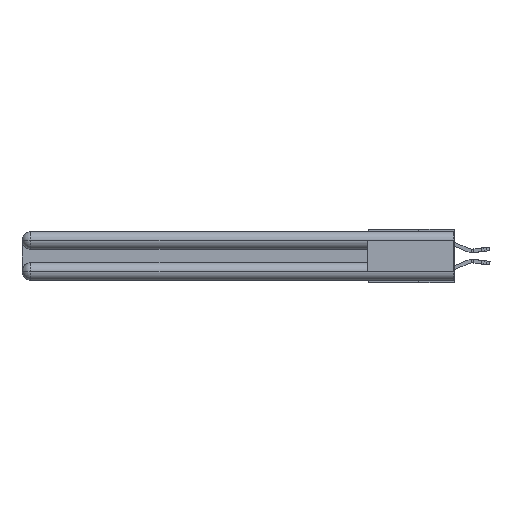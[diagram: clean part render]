
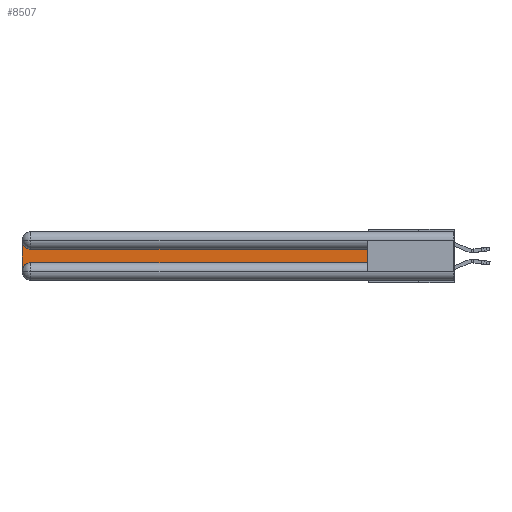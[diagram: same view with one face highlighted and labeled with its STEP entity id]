
A CAD part, left-side view. The second image highlights one B-rep face of the part: STEP entity #8507.
In plain terms, the highlighted planar face has unit normal (-1, 0, 0).
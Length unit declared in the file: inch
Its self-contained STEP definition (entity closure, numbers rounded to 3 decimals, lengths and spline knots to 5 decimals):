
#123 = CARTESIAN_POINT ( 'NONE',  ( 0.075, 3., -0.2175 ) ) ;
#2164 = LINE ( 'NONE', #10606, #26529 ) ;
#2321 = FACE_OUTER_BOUND ( 'NONE', #27542, .T. ) ;
#2388 = ORIENTED_EDGE ( 'NONE', *, *, #28134, .T. ) ;
#3236 = LINE ( 'NONE', #13092, #13530 ) ;
#3814 = CARTESIAN_POINT ( 'NONE',  ( 0.075, 2.94, -0.2775 ) ) ;
#4201 = EDGE_CURVE ( 'NONE', #28403, #14134, #21921, .T. ) ;
#6936 = CARTESIAN_POINT ( 'NONE',  ( 0.075, 2.94, -0.0625 ) ) ;
#6988 = AXIS2_PLACEMENT_3D ( 'NONE', #6936, #8967, #22307 ) ;
#7721 = ORIENTED_EDGE ( 'NONE', *, *, #15233, .T. ) ;
#8307 = VERTEX_POINT ( 'NONE', #20167 ) ;
#8507 = ADVANCED_FACE ( 'NONE', ( #2321 ), #12040, .F. ) ;
#8967 = DIRECTION ( 'NONE',  ( 1., 0., 0. ) ) ;
#9269 = AXIS2_PLACEMENT_3D ( 'NONE', #10018, #27425, #23078 ) ;
#10018 = CARTESIAN_POINT ( 'NONE',  ( 0.075, 3., -0.1225 ) ) ;
#10606 = CARTESIAN_POINT ( 'NONE',  ( 0.075, 0.6, -0.1225 ) ) ;
#11054 = CARTESIAN_POINT ( 'NONE',  ( 0.075, 0.6, -0.1225 ) ) ;
#12040 = PLANE ( 'NONE',  #9269 ) ;
#12139 = DIRECTION ( 'NONE',  ( 0., 0., 1. ) ) ;
#13092 = CARTESIAN_POINT ( 'NONE',  ( 0.075, 0.6, -0.2175 ) ) ;
#13530 = VECTOR ( 'NONE', #26231, 39.37008 ) ;
#13618 = ORIENTED_EDGE ( 'NONE', *, *, #28012, .T. ) ;
#14134 = VERTEX_POINT ( 'NONE', #11054 ) ;
#15233 = EDGE_CURVE ( 'NONE', #26937, #8307, #15254, .T. ) ;
#15254 = LINE ( 'NONE', #123, #21451 ) ;
#16101 = VECTOR ( 'NONE', #12139, 39.37008 ) ;
#16615 = DIRECTION ( 'NONE',  ( 1., 0., 0. ) ) ;
#17108 = ORIENTED_EDGE ( 'NONE', *, *, #18627, .T. ) ;
#17190 = CARTESIAN_POINT ( 'NONE',  ( 0.075, 0.6, -0.2175 ) ) ;
#17533 = VERTEX_POINT ( 'NONE', #18312 ) ;
#17835 = CIRCLE ( 'NONE', #24582, 0.06 ) ;
#18312 = CARTESIAN_POINT ( 'NONE',  ( 0.075, 2.94, -0.1225 ) ) ;
#18627 = EDGE_CURVE ( 'NONE', #14134, #17533, #2164, .T. ) ;
#18814 = ORIENTED_EDGE ( 'NONE', *, *, #4201, .T. ) ;
#20167 = CARTESIAN_POINT ( 'NONE',  ( 0.075, 3., -0.2775 ) ) ;
#21005 = DIRECTION ( 'NONE',  ( 0., 0., -1. ) ) ;
#21451 = VECTOR ( 'NONE', #22004, 39.37008 ) ;
#21921 = LINE ( 'NONE', #17190, #16101 ) ;
#22004 = DIRECTION ( 'NONE',  ( 0., 0., -1. ) ) ;
#22307 = DIRECTION ( 'NONE',  ( 0., 0., -1. ) ) ;
#22406 = VERTEX_POINT ( 'NONE', #24631 ) ;
#22984 = EDGE_CURVE ( 'NONE', #8307, #22406, #17835, .T. ) ;
#23078 = DIRECTION ( 'NONE',  ( 0., 0., -1. ) ) ;
#23927 = CARTESIAN_POINT ( 'NONE',  ( 0.075, 3., -0.0625 ) ) ;
#24182 = CIRCLE ( 'NONE', #6988, 0.06 ) ;
#24582 = AXIS2_PLACEMENT_3D ( 'NONE', #3814, #16615, #21005 ) ;
#24631 = CARTESIAN_POINT ( 'NONE',  ( 0.075, 2.94, -0.2175 ) ) ;
#26231 = DIRECTION ( 'NONE',  ( 0., -1., 0. ) ) ;
#26529 = VECTOR ( 'NONE', #28377, 39.37008 ) ;
#26937 = VERTEX_POINT ( 'NONE', #23927 ) ;
#27425 = DIRECTION ( 'NONE',  ( 1., 0., 0. ) ) ;
#27542 = EDGE_LOOP ( 'NONE', ( #17108, #2388, #7721, #28202, #13618, #18814 ) ) ;
#27881 = CARTESIAN_POINT ( 'NONE',  ( 0.075, 0.6, -0.2175 ) ) ;
#28012 = EDGE_CURVE ( 'NONE', #22406, #28403, #3236, .T. ) ;
#28134 = EDGE_CURVE ( 'NONE', #17533, #26937, #24182, .T. ) ;
#28202 = ORIENTED_EDGE ( 'NONE', *, *, #22984, .T. ) ;
#28377 = DIRECTION ( 'NONE',  ( 0., 1., 0. ) ) ;
#28403 = VERTEX_POINT ( 'NONE', #27881 ) ;
